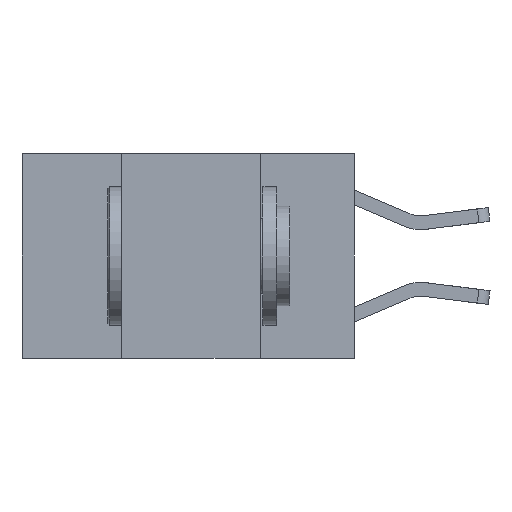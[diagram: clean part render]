
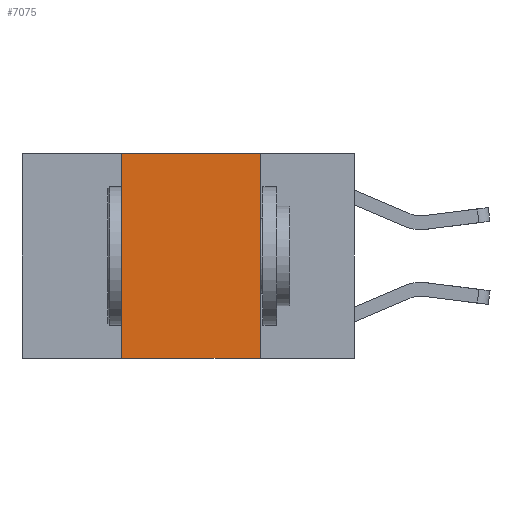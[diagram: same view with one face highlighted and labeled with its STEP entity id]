
A CAD part, left-side view. The second image highlights one B-rep face of the part: STEP entity #7075.
In plain terms, the highlighted planar face has unit normal (-1, 0, 0).
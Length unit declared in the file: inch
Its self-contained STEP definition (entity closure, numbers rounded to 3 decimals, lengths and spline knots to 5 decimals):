
#283 = VERTEX_POINT ( 'NONE', #2603 ) ;
#389 = EDGE_CURVE ( 'NONE', #852, #3810, #7016, .T. ) ;
#403 = CARTESIAN_POINT ( 'NONE',  ( 0., 0.17, 0. ) ) ;
#638 = VECTOR ( 'NONE', #4233, 39.37008 ) ;
#852 = VERTEX_POINT ( 'NONE', #2743 ) ;
#1193 = DIRECTION ( 'NONE',  ( 0., 0., -1. ) ) ;
#1510 = AXIS2_PLACEMENT_3D ( 'NONE', #2739, #8877, #4249 ) ;
#2410 = ORIENTED_EDGE ( 'NONE', *, *, #9573, .F. ) ;
#2547 = CARTESIAN_POINT ( 'NONE',  ( 0., 0.42, 0. ) ) ;
#2603 = CARTESIAN_POINT ( 'NONE',  ( 0., 0.17, -0.37 ) ) ;
#2739 = CARTESIAN_POINT ( 'NONE',  ( 0., 0.6, 0. ) ) ;
#2743 = CARTESIAN_POINT ( 'NONE',  ( 0., 0.42, -0.37 ) ) ;
#2765 = ORIENTED_EDGE ( 'NONE', *, *, #4296, .F. ) ;
#3108 = VECTOR ( 'NONE', #5750, 39.37008 ) ;
#3654 = EDGE_LOOP ( 'NONE', ( #2410, #2765, #4441, #4588 ) ) ;
#3810 = VERTEX_POINT ( 'NONE', #9800 ) ;
#3955 = EDGE_CURVE ( 'NONE', #852, #283, #6253, .T. ) ;
#3986 = FACE_OUTER_BOUND ( 'NONE', #3654, .T. ) ;
#4157 = VECTOR ( 'NONE', #8583, 39.37008 ) ;
#4233 = DIRECTION ( 'NONE',  ( 0., 0., 1. ) ) ;
#4249 = DIRECTION ( 'NONE',  ( 0., 0., -1. ) ) ;
#4296 = EDGE_CURVE ( 'NONE', #3810, #7183, #9222, .T. ) ;
#4441 = ORIENTED_EDGE ( 'NONE', *, *, #389, .F. ) ;
#4588 = ORIENTED_EDGE ( 'NONE', *, *, #3955, .T. ) ;
#5238 = VECTOR ( 'NONE', #1193, 39.37008 ) ;
#5491 = LINE ( 'NONE', #403, #5238 ) ;
#5750 = DIRECTION ( 'NONE',  ( 0., -1., 0. ) ) ;
#5960 = CARTESIAN_POINT ( 'NONE',  ( 0., 0.6, 0. ) ) ;
#6253 = LINE ( 'NONE', #8647, #4157 ) ;
#7016 = LINE ( 'NONE', #2547, #638 ) ;
#7075 = ADVANCED_FACE ( 'NONE', ( #3986 ), #8134, .F. ) ;
#7183 = VERTEX_POINT ( 'NONE', #9741 ) ;
#8134 = PLANE ( 'NONE',  #1510 ) ;
#8583 = DIRECTION ( 'NONE',  ( 0., -1., 0. ) ) ;
#8647 = CARTESIAN_POINT ( 'NONE',  ( 0., 0.6, -0.37 ) ) ;
#8877 = DIRECTION ( 'NONE',  ( 1., 0., 0. ) ) ;
#9222 = LINE ( 'NONE', #5960, #3108 ) ;
#9573 = EDGE_CURVE ( 'NONE', #7183, #283, #5491, .T. ) ;
#9741 = CARTESIAN_POINT ( 'NONE',  ( 0., 0.17, 0. ) ) ;
#9800 = CARTESIAN_POINT ( 'NONE',  ( 0., 0.42, 0. ) ) ;
